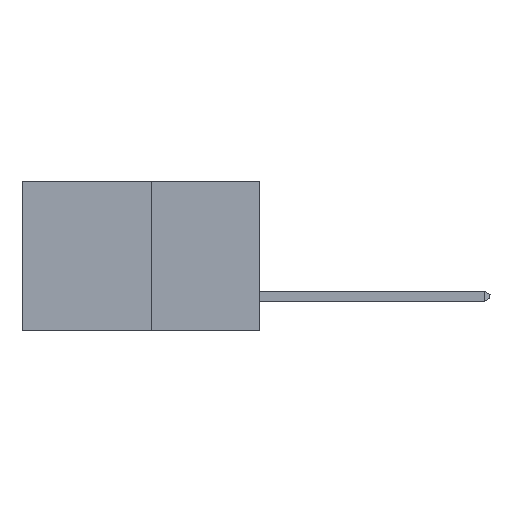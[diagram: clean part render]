
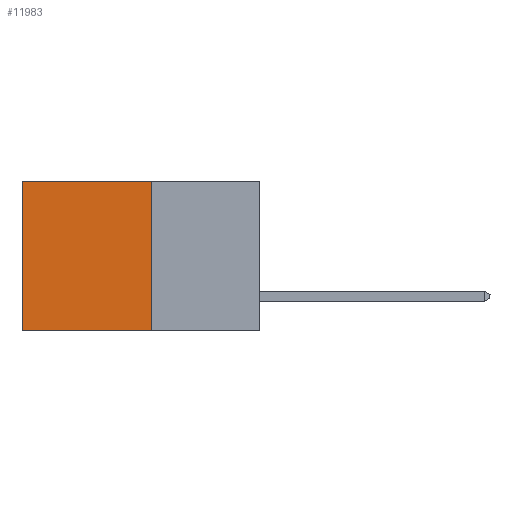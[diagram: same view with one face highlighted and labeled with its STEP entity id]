
A CAD part, left-side view. The second image highlights one B-rep face of the part: STEP entity #11983.
In plain terms, the highlighted planar face has unit normal (-1, 0, 0).
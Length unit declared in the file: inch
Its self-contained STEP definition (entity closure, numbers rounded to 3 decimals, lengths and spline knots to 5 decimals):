
#462 = VERTEX_POINT ( 'NONE', #9030 ) ;
#517 = EDGE_CURVE ( 'NONE', #462, #11885, #12013, .T. ) ;
#1042 = VECTOR ( 'NONE', #4680, 39.37008 ) ;
#1305 = CARTESIAN_POINT ( 'NONE',  ( 0.277, 0.59, 0. ) ) ;
#1504 = VERTEX_POINT ( 'NONE', #4151 ) ;
#1711 = PLANE ( 'NONE',  #1837 ) ;
#1837 = AXIS2_PLACEMENT_3D ( 'NONE', #9200, #3602, #10097 ) ;
#1878 = ORIENTED_EDGE ( 'NONE', *, *, #8445, .T. ) ;
#2059 = EDGE_LOOP ( 'NONE', ( #1878, #2192, #2256, #2309 ) ) ;
#2177 = CARTESIAN_POINT ( 'NONE',  ( 0.277, 0.59, -0.37 ) ) ;
#2192 = ORIENTED_EDGE ( 'NONE', *, *, #517, .F. ) ;
#2256 = ORIENTED_EDGE ( 'NONE', *, *, #8208, .F. ) ;
#2309 = ORIENTED_EDGE ( 'NONE', *, *, #7890, .T. ) ;
#2645 = CARTESIAN_POINT ( 'NONE',  ( 0.277, 0.27, -0.37 ) ) ;
#3287 = VERTEX_POINT ( 'NONE', #1305 ) ;
#3304 = LINE ( 'NONE', #4647, #1042 ) ;
#3602 = DIRECTION ( 'NONE',  ( 1., 0., 0. ) ) ;
#4056 = LINE ( 'NONE', #9053, #11118 ) ;
#4071 = DIRECTION ( 'NONE',  ( 0., 0., -1. ) ) ;
#4151 = CARTESIAN_POINT ( 'NONE',  ( 0.277, 0.27, 0. ) ) ;
#4647 = CARTESIAN_POINT ( 'NONE',  ( 0.277, 0.27, -0.37 ) ) ;
#4680 = DIRECTION ( 'NONE',  ( 0., 0., -1. ) ) ;
#5370 = VECTOR ( 'NONE', #8991, 39.37008 ) ;
#5396 = VECTOR ( 'NONE', #4071, 39.37008 ) ;
#7890 = EDGE_CURVE ( 'NONE', #1504, #3287, #4056, .T. ) ;
#8208 = EDGE_CURVE ( 'NONE', #1504, #462, #3304, .T. ) ;
#8445 = EDGE_CURVE ( 'NONE', #3287, #11885, #10265, .T. ) ;
#8991 = DIRECTION ( 'NONE',  ( 0., 1., 0. ) ) ;
#9030 = CARTESIAN_POINT ( 'NONE',  ( 0.277, 0.27, -0.37 ) ) ;
#9033 = DIRECTION ( 'NONE',  ( 0., 1., 0. ) ) ;
#9053 = CARTESIAN_POINT ( 'NONE',  ( 0.277, 0.27, 0. ) ) ;
#9200 = CARTESIAN_POINT ( 'NONE',  ( 0.277, 0.27, -0.37 ) ) ;
#9897 = CARTESIAN_POINT ( 'NONE',  ( 0.277, 0.59, -0.37 ) ) ;
#10097 = DIRECTION ( 'NONE',  ( 0., 0., -1. ) ) ;
#10265 = LINE ( 'NONE', #2177, #5396 ) ;
#11118 = VECTOR ( 'NONE', #9033, 39.37008 ) ;
#11435 = FACE_OUTER_BOUND ( 'NONE', #2059, .T. ) ;
#11885 = VERTEX_POINT ( 'NONE', #9897 ) ;
#11983 = ADVANCED_FACE ( 'NONE', ( #11435 ), #1711, .F. ) ;
#12013 = LINE ( 'NONE', #2645, #5370 ) ;
